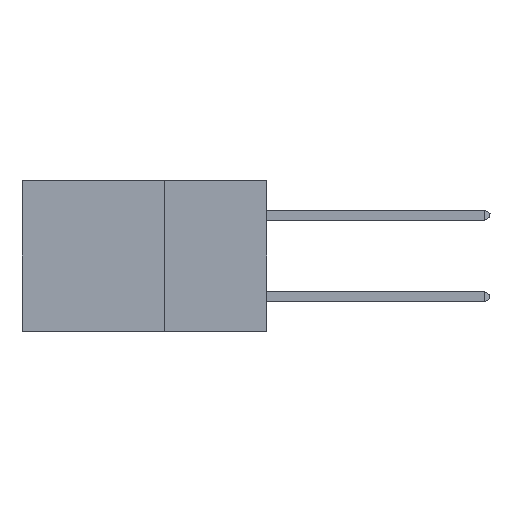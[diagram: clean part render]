
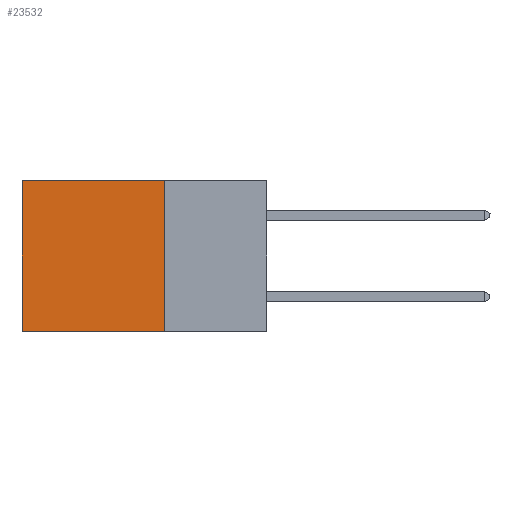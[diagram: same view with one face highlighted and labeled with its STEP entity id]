
A CAD part, left-side view. The second image highlights one B-rep face of the part: STEP entity #23532.
In plain terms, the highlighted planar face has unit normal (-1, 0, 0).
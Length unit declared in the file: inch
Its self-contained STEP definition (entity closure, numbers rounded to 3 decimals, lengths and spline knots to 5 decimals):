
#1197 = CARTESIAN_POINT ( 'NONE',  ( 0.2875, 0.25, 0. ) ) ;
#1919 = CARTESIAN_POINT ( 'NONE',  ( 0.2875, 0.6, -0.37 ) ) ;
#2789 = EDGE_CURVE ( 'NONE', #20705, #18608, #13941, .T. ) ;
#3088 = DIRECTION ( 'NONE',  ( 0., 1., 0. ) ) ;
#3226 = VECTOR ( 'NONE', #5283, 39.37008 ) ;
#3437 = CARTESIAN_POINT ( 'NONE',  ( 0.2875, 0.25, -0.37 ) ) ;
#4207 = DIRECTION ( 'NONE',  ( 0., 1., 0. ) ) ;
#5283 = DIRECTION ( 'NONE',  ( 0., 0., -1. ) ) ;
#7206 = ORIENTED_EDGE ( 'NONE', *, *, #15036, .F. ) ;
#8288 = VECTOR ( 'NONE', #20771, 39.37008 ) ;
#8797 = DIRECTION ( 'NONE',  ( 0., 0., -1. ) ) ;
#9560 = EDGE_CURVE ( 'NONE', #18608, #17481, #10934, .T. ) ;
#10934 = LINE ( 'NONE', #16508, #8288 ) ;
#11211 = LINE ( 'NONE', #11335, #3226 ) ;
#11335 = CARTESIAN_POINT ( 'NONE',  ( 0.2875, 0.25, 0. ) ) ;
#11919 = AXIS2_PLACEMENT_3D ( 'NONE', #1197, #23834, #8797 ) ;
#12683 = LINE ( 'NONE', #20397, #13692 ) ;
#12892 = CARTESIAN_POINT ( 'NONE',  ( 0.2875, 0.25, 0. ) ) ;
#13692 = VECTOR ( 'NONE', #3088, 39.37008 ) ;
#13941 = LINE ( 'NONE', #23919, #19291 ) ;
#14600 = CARTESIAN_POINT ( 'NONE',  ( 0.2875, 0.6, 0. ) ) ;
#14906 = ORIENTED_EDGE ( 'NONE', *, *, #15989, .F. ) ;
#15036 = EDGE_CURVE ( 'NONE', #20705, #24060, #11211, .T. ) ;
#15989 = EDGE_CURVE ( 'NONE', #24060, #17481, #12683, .T. ) ;
#16508 = CARTESIAN_POINT ( 'NONE',  ( 0.2875, 0.6, 0. ) ) ;
#17481 = VERTEX_POINT ( 'NONE', #1919 ) ;
#17720 = ORIENTED_EDGE ( 'NONE', *, *, #2789, .T. ) ;
#18392 = PLANE ( 'NONE',  #11919 ) ;
#18393 = ORIENTED_EDGE ( 'NONE', *, *, #9560, .T. ) ;
#18608 = VERTEX_POINT ( 'NONE', #14600 ) ;
#19291 = VECTOR ( 'NONE', #4207, 39.37008 ) ;
#20168 = FACE_OUTER_BOUND ( 'NONE', #24771, .T. ) ;
#20397 = CARTESIAN_POINT ( 'NONE',  ( 0.2875, 0.25, -0.37 ) ) ;
#20705 = VERTEX_POINT ( 'NONE', #12892 ) ;
#20771 = DIRECTION ( 'NONE',  ( 0., 0., -1. ) ) ;
#23532 = ADVANCED_FACE ( 'NONE', ( #20168 ), #18392, .F. ) ;
#23834 = DIRECTION ( 'NONE',  ( 1., 0., 0. ) ) ;
#23919 = CARTESIAN_POINT ( 'NONE',  ( 0.2875, 0.25, 0. ) ) ;
#24060 = VERTEX_POINT ( 'NONE', #3437 ) ;
#24771 = EDGE_LOOP ( 'NONE', ( #18393, #14906, #7206, #17720 ) ) ;
